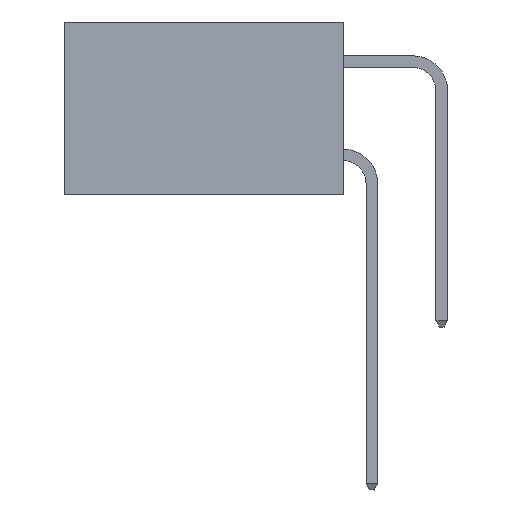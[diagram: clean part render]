
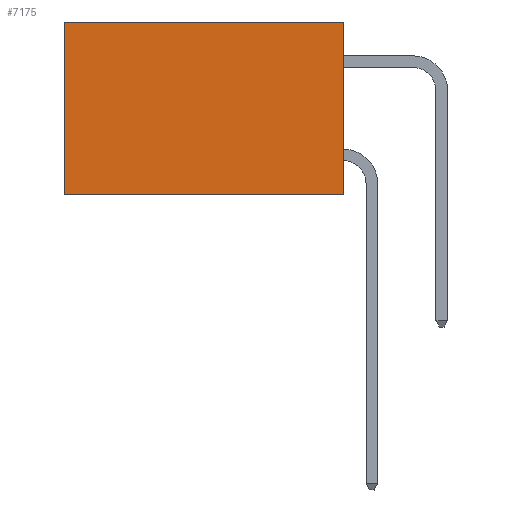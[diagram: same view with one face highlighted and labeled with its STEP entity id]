
A CAD part, left-side view. The second image highlights one B-rep face of the part: STEP entity #7175.
In plain terms, the highlighted planar face has unit normal (-1, 0, 0).
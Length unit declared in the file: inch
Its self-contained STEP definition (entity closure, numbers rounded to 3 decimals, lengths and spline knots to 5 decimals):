
#62 = CARTESIAN_POINT ( 'NONE',  ( 0.2615, 0., -0.37 ) ) ;
#219 = LINE ( 'NONE', #62, #2474 ) ;
#242 = VERTEX_POINT ( 'NONE', #13388 ) ;
#1157 = VERTEX_POINT ( 'NONE', #1872 ) ;
#1262 = VECTOR ( 'NONE', #4319, 39.37008 ) ;
#1289 = DIRECTION ( 'NONE',  ( 0., 0., -1. ) ) ;
#1872 = CARTESIAN_POINT ( 'NONE',  ( 0.2615, 0., -0.37 ) ) ;
#1973 = PLANE ( 'NONE',  #8024 ) ;
#2474 = VECTOR ( 'NONE', #1289, 39.37008 ) ;
#3411 = CARTESIAN_POINT ( 'NONE',  ( 0.2615, 0., 0. ) ) ;
#4319 = DIRECTION ( 'NONE',  ( 0., 1., 0. ) ) ;
#4333 = VECTOR ( 'NONE', #5226, 39.37008 ) ;
#4473 = CARTESIAN_POINT ( 'NONE',  ( 0.2615, 0.6, -0.37 ) ) ;
#4808 = CARTESIAN_POINT ( 'NONE',  ( 0.2615, 0.6, -0.37 ) ) ;
#5226 = DIRECTION ( 'NONE',  ( 0., 1., 0. ) ) ;
#5604 = EDGE_CURVE ( 'NONE', #13523, #1157, #219, .T. ) ;
#6626 = EDGE_CURVE ( 'NONE', #1157, #8741, #14612, .T. ) ;
#6669 = CARTESIAN_POINT ( 'NONE',  ( 0.2615, 0., -0.37 ) ) ;
#7175 = ADVANCED_FACE ( 'NONE', ( #12516 ), #1973, .F. ) ;
#7613 = CARTESIAN_POINT ( 'NONE',  ( 0.2615, 0., -0.37 ) ) ;
#7885 = ORIENTED_EDGE ( 'NONE', *, *, #13825, .T. ) ;
#8008 = LINE ( 'NONE', #14873, #1262 ) ;
#8024 = AXIS2_PLACEMENT_3D ( 'NONE', #6669, #9899, #14597 ) ;
#8145 = ORIENTED_EDGE ( 'NONE', *, *, #6626, .F. ) ;
#8741 = VERTEX_POINT ( 'NONE', #4808 ) ;
#9093 = EDGE_CURVE ( 'NONE', #242, #8741, #10249, .T. ) ;
#9899 = DIRECTION ( 'NONE',  ( 1., 0., 0. ) ) ;
#9996 = EDGE_LOOP ( 'NONE', ( #13438, #8145, #12673, #7885 ) ) ;
#10249 = LINE ( 'NONE', #4473, #10788 ) ;
#10788 = VECTOR ( 'NONE', #14958, 39.37008 ) ;
#12516 = FACE_OUTER_BOUND ( 'NONE', #9996, .T. ) ;
#12673 = ORIENTED_EDGE ( 'NONE', *, *, #5604, .F. ) ;
#13388 = CARTESIAN_POINT ( 'NONE',  ( 0.2615, 0.6, 0. ) ) ;
#13438 = ORIENTED_EDGE ( 'NONE', *, *, #9093, .T. ) ;
#13523 = VERTEX_POINT ( 'NONE', #3411 ) ;
#13825 = EDGE_CURVE ( 'NONE', #13523, #242, #8008, .T. ) ;
#14597 = DIRECTION ( 'NONE',  ( 0., 0., -1. ) ) ;
#14612 = LINE ( 'NONE', #7613, #4333 ) ;
#14873 = CARTESIAN_POINT ( 'NONE',  ( 0.2615, 0., 0. ) ) ;
#14958 = DIRECTION ( 'NONE',  ( 0., 0., -1. ) ) ;
